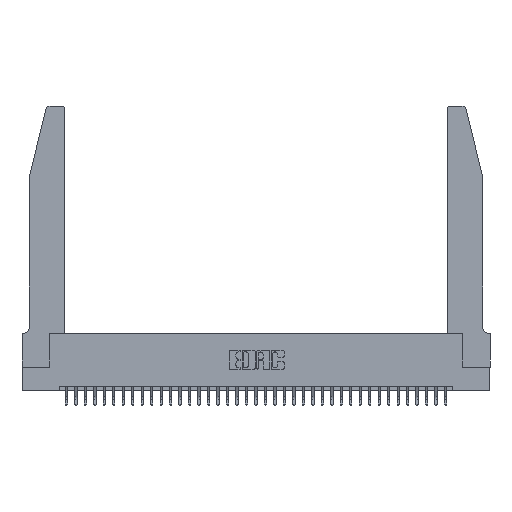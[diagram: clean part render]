
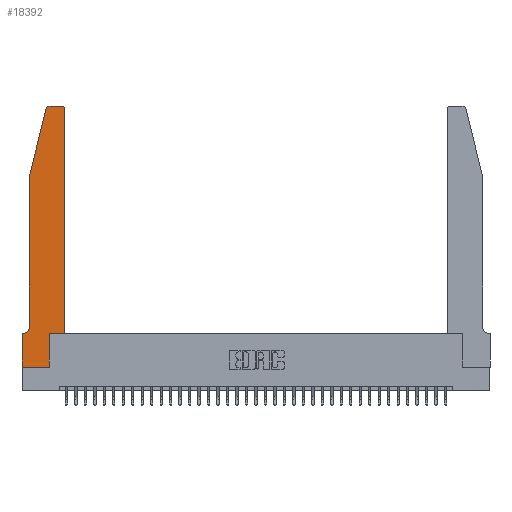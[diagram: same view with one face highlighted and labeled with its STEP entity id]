
A CAD part, top view. The second image highlights one B-rep face of the part: STEP entity #18392.
In plain terms, the highlighted planar face has unit normal (0, 0, 1).
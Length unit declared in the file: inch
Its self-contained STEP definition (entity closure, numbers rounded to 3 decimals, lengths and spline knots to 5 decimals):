
#139 = CARTESIAN_POINT ( 'NONE',  ( 0.4205, 2.75, 0.37 ) ) ;
#193 = VERTEX_POINT ( 'NONE', #21803 ) ;
#418 = EDGE_CURVE ( 'NONE', #34136, #21438, #26459, .T. ) ;
#439 = CARTESIAN_POINT ( 'NONE',  ( 0.2865, 0.35, 0.37 ) ) ;
#1104 = CARTESIAN_POINT ( 'NONE',  ( 0.0755, 2., 0.37 ) ) ;
#1381 = CARTESIAN_POINT ( 'NONE',  ( 0., 0., 0.37 ) ) ;
#1729 = VERTEX_POINT ( 'NONE', #1762 ) ;
#1762 = CARTESIAN_POINT ( 'NONE',  ( 0., 0., 0.37 ) ) ;
#1826 = DIRECTION ( 'NONE',  ( 1., 0., 0. ) ) ;
#1930 = CIRCLE ( 'NONE', #36680, 0.03 ) ;
#2450 = FACE_OUTER_BOUND ( 'NONE', #33783, .T. ) ;
#2531 = EDGE_CURVE ( 'NONE', #21324, #18966, #26752, .T. ) ;
#2680 = ORIENTED_EDGE ( 'NONE', *, *, #21565, .T. ) ;
#2773 = CARTESIAN_POINT ( 'NONE',  ( 0.4205, 2.72, 0.37 ) ) ;
#3000 = CARTESIAN_POINT ( 'NONE',  ( 0.2605, 2.75, 0.37 ) ) ;
#3273 = LINE ( 'NONE', #16358, #22322 ) ;
#3549 = VECTOR ( 'NONE', #4043, 39.37008 ) ;
#4043 = DIRECTION ( 'NONE',  ( 0., -1., 0. ) ) ;
#4332 = DIRECTION ( 'NONE',  ( 0., -1., 0. ) ) ;
#4355 = DIRECTION ( 'NONE',  ( -1., 0., 0. ) ) ;
#4395 = ORIENTED_EDGE ( 'NONE', *, *, #12366, .T. ) ;
#4756 = CARTESIAN_POINT ( 'NONE',  ( 0.2865, 0.35, 0.37 ) ) ;
#4920 = ORIENTED_EDGE ( 'NONE', *, *, #5761, .T. ) ;
#5215 = CARTESIAN_POINT ( 'NONE',  ( 0.284, 2.75, 0.37 ) ) ;
#5456 = VECTOR ( 'NONE', #9329, 39.37008 ) ;
#5761 = EDGE_CURVE ( 'NONE', #6603, #11838, #8777, .T. ) ;
#5959 = VERTEX_POINT ( 'NONE', #5215 ) ;
#6603 = VERTEX_POINT ( 'NONE', #13850 ) ;
#6826 = ORIENTED_EDGE ( 'NONE', *, *, #2531, .T. ) ;
#6948 = EDGE_CURVE ( 'NONE', #193, #21324, #9153, .T. ) ;
#7232 = EDGE_CURVE ( 'NONE', #37303, #30547, #3273, .T. ) ;
#7443 = AXIS2_PLACEMENT_3D ( 'NONE', #12620, #32788, #15529 ) ;
#7698 = DIRECTION ( 'NONE',  ( 0., 1., 0. ) ) ;
#7933 = CARTESIAN_POINT ( 'NONE',  ( 0.0755, 2., 0.37 ) ) ;
#8234 = VECTOR ( 'NONE', #15226, 39.37008 ) ;
#8279 = CARTESIAN_POINT ( 'NONE',  ( 0.0755, 0.42, 0.37 ) ) ;
#8777 = LINE ( 'NONE', #21796, #18387 ) ;
#9153 = LINE ( 'NONE', #29631, #8234 ) ;
#9329 = DIRECTION ( 'NONE',  ( 1., 0., 0. ) ) ;
#9838 = CARTESIAN_POINT ( 'NONE',  ( 0., 0.35, 0.37 ) ) ;
#9841 = ORIENTED_EDGE ( 'NONE', *, *, #35381, .T. ) ;
#9905 = EDGE_CURVE ( 'NONE', #31133, #37303, #11212, .T. ) ;
#10386 = DIRECTION ( 'NONE',  ( 0., 0., 1. ) ) ;
#10827 = CARTESIAN_POINT ( 'NONE',  ( 0.4505, 0.35, 0.37 ) ) ;
#11212 = LINE ( 'NONE', #4756, #25735 ) ;
#11525 = CARTESIAN_POINT ( 'NONE',  ( 0., 0.35, 0.37 ) ) ;
#11650 = ORIENTED_EDGE ( 'NONE', *, *, #418, .T. ) ;
#11651 = PLANE ( 'NONE',  #18668 ) ;
#11838 = VERTEX_POINT ( 'NONE', #9838 ) ;
#12181 = LINE ( 'NONE', #1381, #34224 ) ;
#12259 = CARTESIAN_POINT ( 'NONE',  ( 0., 0., 0.37 ) ) ;
#12366 = EDGE_CURVE ( 'NONE', #30547, #34136, #34759, .T. ) ;
#12620 = CARTESIAN_POINT ( 'NONE',  ( 0.0055, 0.42, 0.37 ) ) ;
#13583 = ORIENTED_EDGE ( 'NONE', *, *, #9905, .T. ) ;
#13850 = CARTESIAN_POINT ( 'NONE',  ( 0.0055, 0.35, 0.37 ) ) ;
#13863 = ORIENTED_EDGE ( 'NONE', *, *, #26479, .T. ) ;
#14071 = VECTOR ( 'NONE', #17534, 39.37008 ) ;
#14132 = LINE ( 'NONE', #12259, #5456 ) ;
#14557 = DIRECTION ( 'NONE',  ( 1., 0., 0. ) ) ;
#15226 = DIRECTION ( 'NONE',  ( -0.239, -0.971, 0. ) ) ;
#15509 = CARTESIAN_POINT ( 'NONE',  ( 0.4505, 0.35, 0.37 ) ) ;
#15529 = DIRECTION ( 'NONE',  ( -1., 0., 0. ) ) ;
#16358 = CARTESIAN_POINT ( 'NONE',  ( 0.4505, 0.35, 0.37 ) ) ;
#17534 = DIRECTION ( 'NONE',  ( -1., 0., 0. ) ) ;
#18387 = VECTOR ( 'NONE', #4355, 39.37008 ) ;
#18392 = ADVANCED_FACE ( 'NONE', ( #2450 ), #11651, .T. ) ;
#18668 = AXIS2_PLACEMENT_3D ( 'NONE', #11525, #31853, #14557 ) ;
#18827 = ORIENTED_EDGE ( 'NONE', *, *, #7232, .T. ) ;
#18966 = VERTEX_POINT ( 'NONE', #8279 ) ;
#21324 = VERTEX_POINT ( 'NONE', #7933 ) ;
#21438 = VERTEX_POINT ( 'NONE', #139 ) ;
#21565 = EDGE_CURVE ( 'NONE', #1729, #31133, #14132, .T. ) ;
#21796 = CARTESIAN_POINT ( 'NONE',  ( 0.0755, 0.35, 0.37 ) ) ;
#21803 = CARTESIAN_POINT ( 'NONE',  ( 0.25487, 2.72718, 0.37 ) ) ;
#21809 = LINE ( 'NONE', #3000, #14071 ) ;
#21966 = CARTESIAN_POINT ( 'NONE',  ( 0.2865, 0., 0.37 ) ) ;
#22322 = VECTOR ( 'NONE', #1826, 39.37008 ) ;
#23492 = CIRCLE ( 'NONE', #7443, 0.07 ) ;
#24960 = DIRECTION ( 'NONE',  ( 1., 0., 0. ) ) ;
#24967 = DIRECTION ( 'NONE',  ( 0., 0., 1. ) ) ;
#25735 = VECTOR ( 'NONE', #7698, 39.37008 ) ;
#26459 = CIRCLE ( 'NONE', #31555, 0.03 ) ;
#26479 = EDGE_CURVE ( 'NONE', #5959, #193, #1930, .T. ) ;
#26752 = LINE ( 'NONE', #1104, #3549 ) ;
#27754 = CARTESIAN_POINT ( 'NONE',  ( 0.284, 2.72, 0.37 ) ) ;
#28165 = VECTOR ( 'NONE', #35532, 39.37008 ) ;
#29631 = CARTESIAN_POINT ( 'NONE',  ( 0.0755, 2., 0.37 ) ) ;
#30298 = EDGE_CURVE ( 'NONE', #18966, #6603, #23492, .T. ) ;
#30547 = VERTEX_POINT ( 'NONE', #10827 ) ;
#30608 = DIRECTION ( 'NONE',  ( 1., 0., 0. ) ) ;
#31133 = VERTEX_POINT ( 'NONE', #21966 ) ;
#31555 = AXIS2_PLACEMENT_3D ( 'NONE', #2773, #24967, #24960 ) ;
#31853 = DIRECTION ( 'NONE',  ( 0., 0., 1. ) ) ;
#32515 = ORIENTED_EDGE ( 'NONE', *, *, #36339, .T. ) ;
#32788 = DIRECTION ( 'NONE',  ( 0., 0., -1. ) ) ;
#33782 = CARTESIAN_POINT ( 'NONE',  ( 0.4505, 2.72, 0.37 ) ) ;
#33783 = EDGE_LOOP ( 'NONE', ( #9841, #13863, #36950, #6826, #36052, #4920, #32515, #2680, #13583, #18827, #4395, #11650 ) ) ;
#34136 = VERTEX_POINT ( 'NONE', #33782 ) ;
#34224 = VECTOR ( 'NONE', #4332, 39.37008 ) ;
#34759 = LINE ( 'NONE', #15509, #28165 ) ;
#35381 = EDGE_CURVE ( 'NONE', #21438, #5959, #21809, .T. ) ;
#35532 = DIRECTION ( 'NONE',  ( 0., 1., 0. ) ) ;
#36052 = ORIENTED_EDGE ( 'NONE', *, *, #30298, .T. ) ;
#36339 = EDGE_CURVE ( 'NONE', #11838, #1729, #12181, .T. ) ;
#36680 = AXIS2_PLACEMENT_3D ( 'NONE', #27754, #10386, #30608 ) ;
#36950 = ORIENTED_EDGE ( 'NONE', *, *, #6948, .T. ) ;
#37303 = VERTEX_POINT ( 'NONE', #439 ) ;
